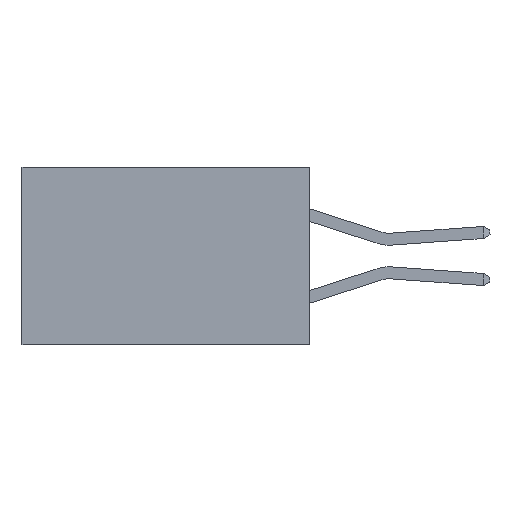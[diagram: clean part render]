
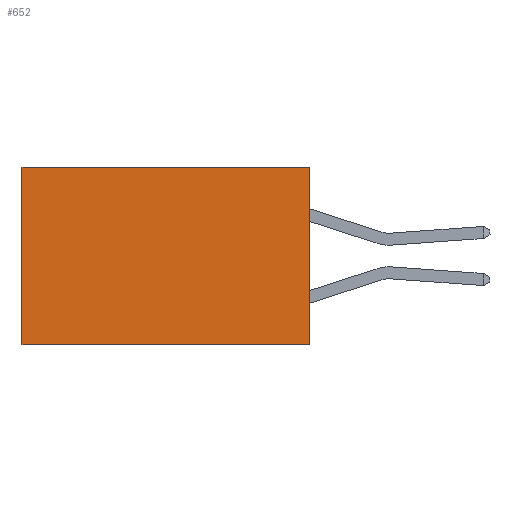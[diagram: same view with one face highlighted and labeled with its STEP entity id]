
A CAD part, left-side view. The second image highlights one B-rep face of the part: STEP entity #652.
In plain terms, the highlighted planar face has unit normal (-1, 0, 0).
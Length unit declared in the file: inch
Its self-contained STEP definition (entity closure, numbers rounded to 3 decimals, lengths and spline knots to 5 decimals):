
#124 = LINE ( 'NONE', #5878, #9689 ) ;
#330 = CARTESIAN_POINT ( 'NONE',  ( 0.298, 0., 0. ) ) ;
#412 = VECTOR ( 'NONE', #2499, 39.37008 ) ;
#644 = CARTESIAN_POINT ( 'NONE',  ( 0.298, 0., 0. ) ) ;
#652 = ADVANCED_FACE ( 'NONE', ( #934 ), #3714, .F. ) ;
#928 = DIRECTION ( 'NONE',  ( 0., 0., -1. ) ) ;
#934 = FACE_OUTER_BOUND ( 'NONE', #3425, .T. ) ;
#1405 = VECTOR ( 'NONE', #4597, 39.37008 ) ;
#1652 = LINE ( 'NONE', #4632, #1405 ) ;
#1818 = CARTESIAN_POINT ( 'NONE',  ( 0.298, 0.6, -0.37 ) ) ;
#1998 = VERTEX_POINT ( 'NONE', #330 ) ;
#2098 = LINE ( 'NONE', #6723, #5846 ) ;
#2499 = DIRECTION ( 'NONE',  ( 0., 0., -1. ) ) ;
#2663 = EDGE_CURVE ( 'NONE', #1998, #6169, #2666, .T. ) ;
#2666 = LINE ( 'NONE', #6397, #412 ) ;
#3425 = EDGE_LOOP ( 'NONE', ( #3634, #4258, #4801, #4307 ) ) ;
#3634 = ORIENTED_EDGE ( 'NONE', *, *, #6262, .T. ) ;
#3714 = PLANE ( 'NONE',  #9671 ) ;
#4258 = ORIENTED_EDGE ( 'NONE', *, *, #9040, .F. ) ;
#4307 = ORIENTED_EDGE ( 'NONE', *, *, #5630, .T. ) ;
#4379 = VERTEX_POINT ( 'NONE', #6742 ) ;
#4597 = DIRECTION ( 'NONE',  ( 0., 1., 0. ) ) ;
#4632 = CARTESIAN_POINT ( 'NONE',  ( 0.298, 0., 0. ) ) ;
#4801 = ORIENTED_EDGE ( 'NONE', *, *, #2663, .F. ) ;
#5287 = DIRECTION ( 'NONE',  ( 1., 0., 0. ) ) ;
#5427 = VERTEX_POINT ( 'NONE', #1818 ) ;
#5630 = EDGE_CURVE ( 'NONE', #1998, #4379, #1652, .T. ) ;
#5846 = VECTOR ( 'NONE', #8561, 39.37008 ) ;
#5878 = CARTESIAN_POINT ( 'NONE',  ( 0.298, 0.6, 0. ) ) ;
#6169 = VERTEX_POINT ( 'NONE', #7031 ) ;
#6262 = EDGE_CURVE ( 'NONE', #4379, #5427, #124, .T. ) ;
#6397 = CARTESIAN_POINT ( 'NONE',  ( 0.298, 0., 0. ) ) ;
#6723 = CARTESIAN_POINT ( 'NONE',  ( 0.298, 0., -0.37 ) ) ;
#6742 = CARTESIAN_POINT ( 'NONE',  ( 0.298, 0.6, 0. ) ) ;
#6983 = DIRECTION ( 'NONE',  ( 0., 0., -1. ) ) ;
#7031 = CARTESIAN_POINT ( 'NONE',  ( 0.298, 0., -0.37 ) ) ;
#8561 = DIRECTION ( 'NONE',  ( 0., 1., 0. ) ) ;
#9040 = EDGE_CURVE ( 'NONE', #6169, #5427, #2098, .T. ) ;
#9671 = AXIS2_PLACEMENT_3D ( 'NONE', #644, #5287, #928 ) ;
#9689 = VECTOR ( 'NONE', #6983, 39.37008 ) ;
